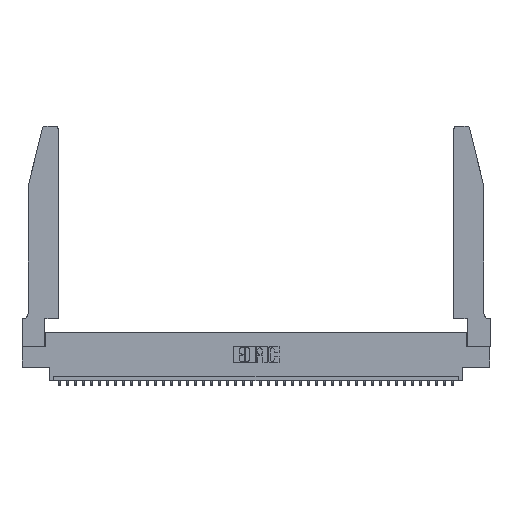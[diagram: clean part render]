
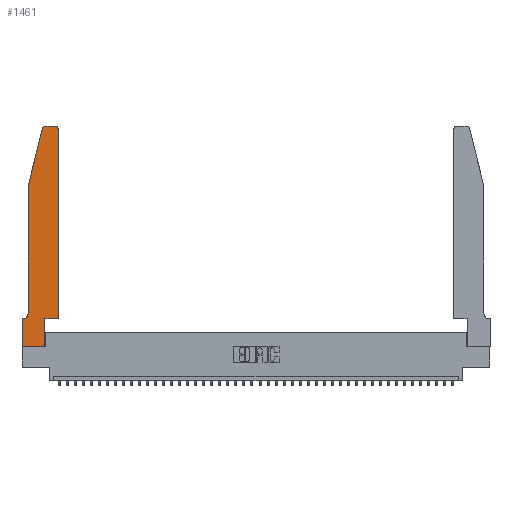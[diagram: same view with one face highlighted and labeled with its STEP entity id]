
A CAD part, top view. The second image highlights one B-rep face of the part: STEP entity #1461.
In plain terms, the highlighted planar face has unit normal (0, 0, 1).
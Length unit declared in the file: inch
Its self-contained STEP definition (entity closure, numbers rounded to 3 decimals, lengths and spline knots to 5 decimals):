
#264 = CARTESIAN_POINT ( 'NONE',  ( 0.4205, 2.75, 0.37 ) ) ;
#421 = EDGE_CURVE ( 'NONE', #25751, #29378, #10583, .T. ) ;
#1015 = VERTEX_POINT ( 'NONE', #26999 ) ;
#1070 = DIRECTION ( 'NONE',  ( 0., 0., 1. ) ) ;
#1375 = CARTESIAN_POINT ( 'NONE',  ( 0., 0.35, 0.37 ) ) ;
#1388 = CARTESIAN_POINT ( 'NONE',  ( 0.4505, 2.72, 0.37 ) ) ;
#1461 = ADVANCED_FACE ( 'NONE', ( #37604 ), #20243, .T. ) ;
#1793 = ORIENTED_EDGE ( 'NONE', *, *, #12795, .T. ) ;
#1859 = EDGE_CURVE ( 'NONE', #36893, #14753, #32027, .T. ) ;
#2241 = LINE ( 'NONE', #4275, #8252 ) ;
#2380 = CARTESIAN_POINT ( 'NONE',  ( 0.0755, 0.42, 0.37 ) ) ;
#3284 = VECTOR ( 'NONE', #23487, 39.37008 ) ;
#3490 = DIRECTION ( 'NONE',  ( -1., 0., 0. ) ) ;
#3551 = CARTESIAN_POINT ( 'NONE',  ( 0.4205, 2.72, 0.37 ) ) ;
#3810 = DIRECTION ( 'NONE',  ( 0., 1., 0. ) ) ;
#3965 = VECTOR ( 'NONE', #9888, 39.37008 ) ;
#4275 = CARTESIAN_POINT ( 'NONE',  ( 0.0755, 2., 0.37 ) ) ;
#4698 = DIRECTION ( 'NONE',  ( 1., 0., 0. ) ) ;
#4819 = ORIENTED_EDGE ( 'NONE', *, *, #25087, .T. ) ;
#5088 = CIRCLE ( 'NONE', #32131, 0.03 ) ;
#6093 = VERTEX_POINT ( 'NONE', #1388 ) ;
#6229 = EDGE_CURVE ( 'NONE', #30929, #28403, #12133, .T. ) ;
#6482 = VECTOR ( 'NONE', #26962, 39.37008 ) ;
#6667 = ORIENTED_EDGE ( 'NONE', *, *, #8111, .T. ) ;
#7060 = CIRCLE ( 'NONE', #32559, 0.03 ) ;
#7507 = DIRECTION ( 'NONE',  ( -0.239, -0.971, 0. ) ) ;
#7661 = ORIENTED_EDGE ( 'NONE', *, *, #421, .T. ) ;
#8111 = EDGE_CURVE ( 'NONE', #17704, #6093, #35447, .T. ) ;
#8252 = VECTOR ( 'NONE', #7507, 39.37008 ) ;
#8685 = VECTOR ( 'NONE', #30270, 39.37008 ) ;
#8849 = VERTEX_POINT ( 'NONE', #17886 ) ;
#9750 = DIRECTION ( 'NONE',  ( 1., 0., 0. ) ) ;
#9888 = DIRECTION ( 'NONE',  ( -1., 0., 0. ) ) ;
#10028 = DIRECTION ( 'NONE',  ( 1., 0., 0. ) ) ;
#10583 = LINE ( 'NONE', #11720, #8685 ) ;
#10707 = CARTESIAN_POINT ( 'NONE',  ( 0.2605, 2.75, 0.37 ) ) ;
#10758 = DIRECTION ( 'NONE',  ( 1., 0., 0. ) ) ;
#11720 = CARTESIAN_POINT ( 'NONE',  ( 0., 0., 0.37 ) ) ;
#12089 = CIRCLE ( 'NONE', #35679, 0.07 ) ;
#12133 = LINE ( 'NONE', #10707, #32089 ) ;
#12795 = EDGE_CURVE ( 'NONE', #14753, #1015, #12089, .T. ) ;
#13610 = ORIENTED_EDGE ( 'NONE', *, *, #21402, .T. ) ;
#13633 = ORIENTED_EDGE ( 'NONE', *, *, #40170, .T. ) ;
#14753 = VERTEX_POINT ( 'NONE', #2380 ) ;
#15070 = LINE ( 'NONE', #31999, #3965 ) ;
#16091 = VERTEX_POINT ( 'NONE', #34006 ) ;
#17113 = CARTESIAN_POINT ( 'NONE',  ( 0.284, 2.72, 0.37 ) ) ;
#17468 = DIRECTION ( 'NONE',  ( 1., 0., 0. ) ) ;
#17704 = VERTEX_POINT ( 'NONE', #39062 ) ;
#17886 = CARTESIAN_POINT ( 'NONE',  ( 0.2865, 0., 0.37 ) ) ;
#19966 = VECTOR ( 'NONE', #9750, 39.37008 ) ;
#20243 = PLANE ( 'NONE',  #41394 ) ;
#20517 = EDGE_CURVE ( 'NONE', #8849, #16091, #29811, .T. ) ;
#21402 = EDGE_CURVE ( 'NONE', #29378, #8849, #35323, .T. ) ;
#23044 = CARTESIAN_POINT ( 'NONE',  ( 0.0055, 0.42, 0.37 ) ) ;
#23339 = CARTESIAN_POINT ( 'NONE',  ( 0.25487, 2.72718, 0.37 ) ) ;
#23487 = DIRECTION ( 'NONE',  ( 0., 1., 0. ) ) ;
#25087 = EDGE_CURVE ( 'NONE', #6093, #30929, #7060, .T. ) ;
#25285 = CARTESIAN_POINT ( 'NONE',  ( 0.4505, 0.35, 0.37 ) ) ;
#25751 = VERTEX_POINT ( 'NONE', #36511 ) ;
#26885 = VECTOR ( 'NONE', #3810, 39.37008 ) ;
#26962 = DIRECTION ( 'NONE',  ( 0., -1., 0. ) ) ;
#26999 = CARTESIAN_POINT ( 'NONE',  ( 0.0055, 0.35, 0.37 ) ) ;
#27592 = LINE ( 'NONE', #25285, #19966 ) ;
#28403 = VERTEX_POINT ( 'NONE', #28454 ) ;
#28454 = CARTESIAN_POINT ( 'NONE',  ( 0.284, 2.75, 0.37 ) ) ;
#28729 = ORIENTED_EDGE ( 'NONE', *, *, #40230, .T. ) ;
#28919 = CARTESIAN_POINT ( 'NONE',  ( 0.0755, 2., 0.37 ) ) ;
#29378 = VERTEX_POINT ( 'NONE', #30696 ) ;
#29771 = VECTOR ( 'NONE', #10758, 39.37008 ) ;
#29811 = LINE ( 'NONE', #39613, #3284 ) ;
#30062 = CARTESIAN_POINT ( 'NONE',  ( 0.0755, 2., 0.37 ) ) ;
#30270 = DIRECTION ( 'NONE',  ( 0., -1., 0. ) ) ;
#30696 = CARTESIAN_POINT ( 'NONE',  ( 0., 0., 0.37 ) ) ;
#30929 = VERTEX_POINT ( 'NONE', #264 ) ;
#31887 = ORIENTED_EDGE ( 'NONE', *, *, #39863, .T. ) ;
#31999 = CARTESIAN_POINT ( 'NONE',  ( 0.0755, 0.35, 0.37 ) ) ;
#32027 = LINE ( 'NONE', #30062, #6482 ) ;
#32089 = VECTOR ( 'NONE', #32934, 39.37008 ) ;
#32131 = AXIS2_PLACEMENT_3D ( 'NONE', #17113, #39843, #4698 ) ;
#32559 = AXIS2_PLACEMENT_3D ( 'NONE', #3551, #32637, #10028 ) ;
#32637 = DIRECTION ( 'NONE',  ( 0., 0., 1. ) ) ;
#32662 = ORIENTED_EDGE ( 'NONE', *, *, #1859, .T. ) ;
#32934 = DIRECTION ( 'NONE',  ( -1., 0., 0. ) ) ;
#33550 = EDGE_LOOP ( 'NONE', ( #35161, #31887, #35685, #32662, #1793, #28729, #7661, #13610, #34976, #13633, #6667, #4819 ) ) ;
#34006 = CARTESIAN_POINT ( 'NONE',  ( 0.2865, 0.35, 0.37 ) ) ;
#34976 = ORIENTED_EDGE ( 'NONE', *, *, #20517, .T. ) ;
#35135 = CARTESIAN_POINT ( 'NONE',  ( 0.4505, 0.35, 0.37 ) ) ;
#35161 = ORIENTED_EDGE ( 'NONE', *, *, #6229, .T. ) ;
#35323 = LINE ( 'NONE', #35531, #29771 ) ;
#35447 = LINE ( 'NONE', #35135, #26885 ) ;
#35531 = CARTESIAN_POINT ( 'NONE',  ( 0., 0., 0.37 ) ) ;
#35679 = AXIS2_PLACEMENT_3D ( 'NONE', #23044, #38770, #3490 ) ;
#35685 = ORIENTED_EDGE ( 'NONE', *, *, #38105, .T. ) ;
#36511 = CARTESIAN_POINT ( 'NONE',  ( 0., 0.35, 0.37 ) ) ;
#36893 = VERTEX_POINT ( 'NONE', #28919 ) ;
#37604 = FACE_OUTER_BOUND ( 'NONE', #33550, .T. ) ;
#38105 = EDGE_CURVE ( 'NONE', #40977, #36893, #2241, .T. ) ;
#38770 = DIRECTION ( 'NONE',  ( 0., 0., -1. ) ) ;
#39062 = CARTESIAN_POINT ( 'NONE',  ( 0.4505, 0.35, 0.37 ) ) ;
#39613 = CARTESIAN_POINT ( 'NONE',  ( 0.2865, 0.35, 0.37 ) ) ;
#39843 = DIRECTION ( 'NONE',  ( 0., 0., 1. ) ) ;
#39863 = EDGE_CURVE ( 'NONE', #28403, #40977, #5088, .T. ) ;
#40170 = EDGE_CURVE ( 'NONE', #16091, #17704, #27592, .T. ) ;
#40230 = EDGE_CURVE ( 'NONE', #1015, #25751, #15070, .T. ) ;
#40977 = VERTEX_POINT ( 'NONE', #23339 ) ;
#41394 = AXIS2_PLACEMENT_3D ( 'NONE', #1375, #1070, #17468 ) ;
